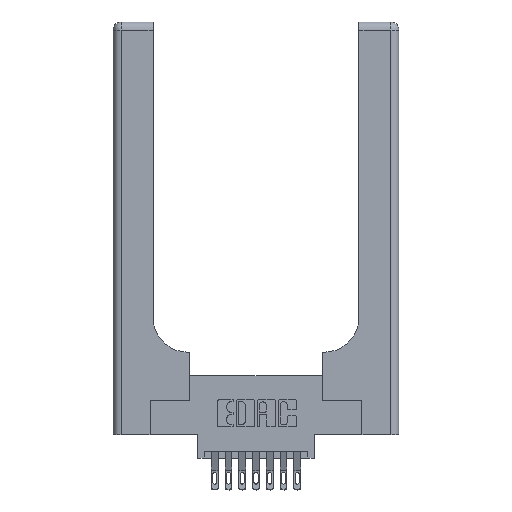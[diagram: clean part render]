
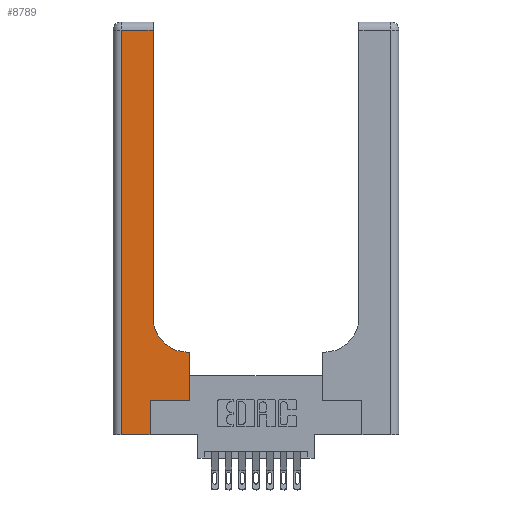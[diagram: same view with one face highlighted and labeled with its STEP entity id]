
A CAD part, top view. The second image highlights one B-rep face of the part: STEP entity #8789.
In plain terms, the highlighted planar face has unit normal (0, 0, 1).
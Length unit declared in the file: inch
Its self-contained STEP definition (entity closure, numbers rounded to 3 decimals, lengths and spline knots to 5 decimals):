
#274 = CARTESIAN_POINT ( 'NONE',  ( 0.5585, 0.25, 0.37 ) ) ;
#293 = EDGE_CURVE ( 'NONE', #10921, #424, #15695, .T. ) ;
#318 = LINE ( 'NONE', #12690, #1099 ) ;
#424 = VERTEX_POINT ( 'NONE', #274 ) ;
#623 = LINE ( 'NONE', #11361, #7453 ) ;
#877 = DIRECTION ( 'NONE',  ( 0., 1., 0. ) ) ;
#970 = VECTOR ( 'NONE', #5142, 39.37008 ) ;
#1099 = VECTOR ( 'NONE', #7853, 39.37008 ) ;
#1137 = CARTESIAN_POINT ( 'NONE',  ( 0.5415, 0.85, 0.37 ) ) ;
#1373 = ORIENTED_EDGE ( 'NONE', *, *, #4699, .T. ) ;
#1691 = EDGE_CURVE ( 'NONE', #10556, #4150, #14708, .T. ) ;
#1882 = AXIS2_PLACEMENT_3D ( 'NONE', #1137, #9627, #13374 ) ;
#2869 = DIRECTION ( 'NONE',  ( 0., 1., 0. ) ) ;
#2916 = PLANE ( 'NONE',  #3256 ) ;
#3256 = AXIS2_PLACEMENT_3D ( 'NONE', #4069, #12674, #13700 ) ;
#3549 = LINE ( 'NONE', #10316, #10171 ) ;
#3874 = CARTESIAN_POINT ( 'NONE',  ( 0.06, 3., 0.37 ) ) ;
#4041 = ORIENTED_EDGE ( 'NONE', *, *, #15579, .T. ) ;
#4065 = CARTESIAN_POINT ( 'NONE',  ( 0.2915, 0.85, 0.37 ) ) ;
#4069 = CARTESIAN_POINT ( 'NONE',  ( 0., 3., 0.37 ) ) ;
#4150 = VERTEX_POINT ( 'NONE', #8165 ) ;
#4171 = ORIENTED_EDGE ( 'NONE', *, *, #13278, .T. ) ;
#4186 = VERTEX_POINT ( 'NONE', #14367 ) ;
#4607 = EDGE_CURVE ( 'NONE', #8839, #10921, #14421, .T. ) ;
#4621 = CARTESIAN_POINT ( 'NONE',  ( 0.5585, 0.25, 0.37 ) ) ;
#4655 = VECTOR ( 'NONE', #2869, 39.37008 ) ;
#4699 = EDGE_CURVE ( 'NONE', #5513, #4186, #11508, .T. ) ;
#4717 = CARTESIAN_POINT ( 'NONE',  ( 0.269, 0.25, 0.37 ) ) ;
#4977 = VERTEX_POINT ( 'NONE', #12033 ) ;
#5042 = ORIENTED_EDGE ( 'NONE', *, *, #4607, .T. ) ;
#5142 = DIRECTION ( 'NONE',  ( 1., 0., 0. ) ) ;
#5227 = ORIENTED_EDGE ( 'NONE', *, *, #293, .T. ) ;
#5482 = EDGE_CURVE ( 'NONE', #4977, #10556, #9201, .T. ) ;
#5513 = VERTEX_POINT ( 'NONE', #9577 ) ;
#5639 = EDGE_LOOP ( 'NONE', ( #13323, #10393, #1373, #4171, #5042, #5227, #4041, #9188, #5959 ) ) ;
#5959 = ORIENTED_EDGE ( 'NONE', *, *, #5482, .T. ) ;
#6925 = CARTESIAN_POINT ( 'NONE',  ( 0.5585, 0.6, 0.37 ) ) ;
#7427 = LINE ( 'NONE', #4621, #8201 ) ;
#7453 = VECTOR ( 'NONE', #13573, 39.37008 ) ;
#7569 = CARTESIAN_POINT ( 'NONE',  ( 0.269, 0.25, 0.37 ) ) ;
#7853 = DIRECTION ( 'NONE',  ( -1., 0., 0. ) ) ;
#7969 = FACE_OUTER_BOUND ( 'NONE', #5639, .T. ) ;
#8137 = CARTESIAN_POINT ( 'NONE',  ( 0.2915, 3., 0.37 ) ) ;
#8165 = CARTESIAN_POINT ( 'NONE',  ( 0.2915, 2.94, 0.37 ) ) ;
#8201 = VECTOR ( 'NONE', #14566, 39.37008 ) ;
#8431 = VECTOR ( 'NONE', #12414, 39.37008 ) ;
#8789 = ADVANCED_FACE ( 'NONE', ( #7969 ), #2916, .F. ) ;
#8839 = VERTEX_POINT ( 'NONE', #11380 ) ;
#9188 = ORIENTED_EDGE ( 'NONE', *, *, #10090, .T. ) ;
#9201 = CIRCLE ( 'NONE', #1882, 0.25 ) ;
#9577 = CARTESIAN_POINT ( 'NONE',  ( 0.06, 2.94, 0.37 ) ) ;
#9627 = DIRECTION ( 'NONE',  ( 0., 0., -1. ) ) ;
#10090 = EDGE_CURVE ( 'NONE', #15508, #4977, #318, .T. ) ;
#10120 = CARTESIAN_POINT ( 'NONE',  ( 0.269, 0., 0.37 ) ) ;
#10171 = VECTOR ( 'NONE', #12721, 39.37008 ) ;
#10316 = CARTESIAN_POINT ( 'NONE',  ( 0., 2.94, 0.37 ) ) ;
#10393 = ORIENTED_EDGE ( 'NONE', *, *, #11039, .T. ) ;
#10556 = VERTEX_POINT ( 'NONE', #4065 ) ;
#10921 = VERTEX_POINT ( 'NONE', #4717 ) ;
#11039 = EDGE_CURVE ( 'NONE', #4150, #5513, #3549, .T. ) ;
#11361 = CARTESIAN_POINT ( 'NONE',  ( 0., 0., 0.37 ) ) ;
#11380 = CARTESIAN_POINT ( 'NONE',  ( 0.269, 0., 0.37 ) ) ;
#11508 = LINE ( 'NONE', #3874, #8431 ) ;
#12033 = CARTESIAN_POINT ( 'NONE',  ( 0.5415, 0.6, 0.37 ) ) ;
#12414 = DIRECTION ( 'NONE',  ( 0., -1., 0. ) ) ;
#12674 = DIRECTION ( 'NONE',  ( 0., 0., -1. ) ) ;
#12690 = CARTESIAN_POINT ( 'NONE',  ( 0.2915, 0.6, 0.37 ) ) ;
#12721 = DIRECTION ( 'NONE',  ( -1., 0., 0. ) ) ;
#13278 = EDGE_CURVE ( 'NONE', #4186, #8839, #623, .T. ) ;
#13323 = ORIENTED_EDGE ( 'NONE', *, *, #1691, .T. ) ;
#13374 = DIRECTION ( 'NONE',  ( 1., 0., 0. ) ) ;
#13573 = DIRECTION ( 'NONE',  ( 1., 0., 0. ) ) ;
#13700 = DIRECTION ( 'NONE',  ( -1., 0., 0. ) ) ;
#14367 = CARTESIAN_POINT ( 'NONE',  ( 0.06, 0., 0.37 ) ) ;
#14421 = LINE ( 'NONE', #10120, #4655 ) ;
#14566 = DIRECTION ( 'NONE',  ( 0., 1., 0. ) ) ;
#14708 = LINE ( 'NONE', #8137, #15279 ) ;
#15279 = VECTOR ( 'NONE', #877, 39.37008 ) ;
#15508 = VERTEX_POINT ( 'NONE', #6925 ) ;
#15579 = EDGE_CURVE ( 'NONE', #424, #15508, #7427, .T. ) ;
#15695 = LINE ( 'NONE', #7569, #970 ) ;
